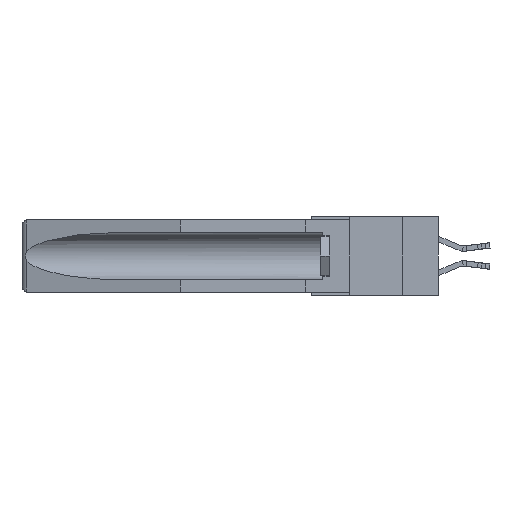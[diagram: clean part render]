
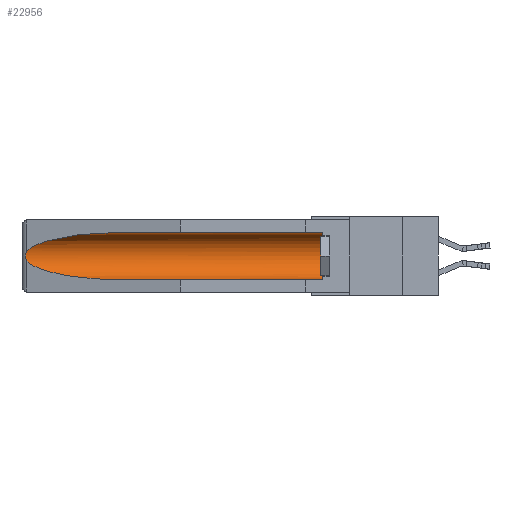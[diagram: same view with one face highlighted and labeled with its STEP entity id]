
A CAD part, left-side view. The second image highlights one B-rep face of the part: STEP entity #22956.
In plain terms, the highlighted cylindrical face has radius 2.857 mm (diameter 5.715 mm), a partial arc.
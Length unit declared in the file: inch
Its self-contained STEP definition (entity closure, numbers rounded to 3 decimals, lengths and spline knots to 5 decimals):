
#512 = CARTESIAN_POINT ( 'NONE',  ( 0.26654, 1.53092, -0.15636 ) ) ;
#1495 = B_SPLINE_CURVE_WITH_KNOTS ( 'NONE', 3,
 ( #16383, #3281, #512, #19023, #21799, #3167, #21676, #3513, #32381, #22036 ),
 .UNSPECIFIED., .F., .F.,
 ( 4, 2, 2, 2, 4 ),
 ( 0., 0.00029, 0.00058, 0.00087, 0.00117 ),
 .UNSPECIFIED. ) ;
#1507 = CARTESIAN_POINT ( 'NONE',  ( 0.155, 0.126, -0.284 ) ) ;
#3167 = CARTESIAN_POINT ( 'NONE',  ( 0.2675, 1.53308, -0.17534 ) ) ;
#3248 = ORIENTED_EDGE ( 'NONE', *, *, #4198, .T. ) ;
#3281 = CARTESIAN_POINT ( 'NONE',  ( 0.26597, 1.52961, -0.15275 ) ) ;
#3391 =( BOUNDED_CURVE ( )  B_SPLINE_CURVE ( 3, ( #12458, #20288, #14993, #14761 ),
 .UNSPECIFIED., .F., .F. ) 
 B_SPLINE_CURVE_WITH_KNOTS ( ( 4, 4 ),
 ( 4.71239, 6.08839 ),
 .UNSPECIFIED. ) 
 CURVE ( )  GEOMETRIC_REPRESENTATION_ITEM ( )  RATIONAL_B_SPLINE_CURVE ( ( 1., 0.848, 0.848, 1. ) ) 
 REPRESENTATION_ITEM ( '' )  );
#3513 = CARTESIAN_POINT ( 'NONE',  ( 0.26655, 1.53094, -0.18657 ) ) ;
#4198 = EDGE_CURVE ( 'NONE', #24264, #15931, #30699, .T. ) ;
#4644 = ORIENTED_EDGE ( 'NONE', *, *, #19632, .T. ) ;
#4700 = ORIENTED_EDGE ( 'NONE', *, *, #30268, .T. ) ;
#4948 = VERTEX_POINT ( 'NONE', #6876 ) ;
#5001 = VECTOR ( 'NONE', #31620, 39.37008 ) ;
#5526 = VERTEX_POINT ( 'NONE', #1507 ) ;
#6672 = CARTESIAN_POINT ( 'NONE',  ( 0.26537, 1.52718, -0.19328 ) ) ;
#6876 = CARTESIAN_POINT ( 'NONE',  ( 0.155, 0.126, -0.059 ) ) ;
#7741 = LINE ( 'NONE', #17487, #27625 ) ;
#8309 = CARTESIAN_POINT ( 'NONE',  ( 0.25451, 1.48313, -0.24835 ) ) ;
#10402 = LINE ( 'NONE', #29444, #5001 ) ;
#10989 = CARTESIAN_POINT ( 'NONE',  ( 0.155, 1.07973, -0.284 ) ) ;
#11816 = AXIS2_PLACEMENT_3D ( 'NONE', #27586, #27694, #30078 ) ;
#12458 = CARTESIAN_POINT ( 'NONE',  ( 0.155, 1.07973, -0.059 ) ) ;
#12667 = VERTEX_POINT ( 'NONE', #12858 ) ;
#12858 = CARTESIAN_POINT ( 'NONE',  ( 0.26537, 1.52718, -0.14972 ) ) ;
#12925 = CARTESIAN_POINT ( 'NONE',  ( 0.155, 0.126, -0.1715 ) ) ;
#14761 = CARTESIAN_POINT ( 'NONE',  ( 0.26537, 1.52718, -0.14972 ) ) ;
#14993 = CARTESIAN_POINT ( 'NONE',  ( 0.25451, 1.48313, -0.09465 ) ) ;
#15931 = VERTEX_POINT ( 'NONE', #20231 ) ;
#16383 = CARTESIAN_POINT ( 'NONE',  ( 0.26537, 1.52718, -0.14972 ) ) ;
#16407 = CARTESIAN_POINT ( 'NONE',  ( 0.21114, 1.30732, -0.284 ) ) ;
#16977 = EDGE_CURVE ( 'NONE', #5526, #15931, #10402, .T. ) ;
#17487 = CARTESIAN_POINT ( 'NONE',  ( 0.155, -0.30754, -0.059 ) ) ;
#19023 = CARTESIAN_POINT ( 'NONE',  ( 0.2673, 1.5327, -0.16383 ) ) ;
#19632 = EDGE_CURVE ( 'NONE', #4948, #30372, #7741, .T. ) ;
#20231 = CARTESIAN_POINT ( 'NONE',  ( 0.155, 1.07973, -0.284 ) ) ;
#20288 = CARTESIAN_POINT ( 'NONE',  ( 0.21114, 1.30732, -0.059 ) ) ;
#21014 = AXIS2_PLACEMENT_3D ( 'NONE', #12925, #26079, #31247 ) ;
#21676 = CARTESIAN_POINT ( 'NONE',  ( 0.2673, 1.53269, -0.17917 ) ) ;
#21703 = CARTESIAN_POINT ( 'NONE',  ( 0.26537, 1.52718, -0.19328 ) ) ;
#21799 = CARTESIAN_POINT ( 'NONE',  ( 0.2675, 1.53308, -0.16763 ) ) ;
#22036 = CARTESIAN_POINT ( 'NONE',  ( 0.26537, 1.52718, -0.19328 ) ) ;
#22956 = ADVANCED_FACE ( 'NONE', ( #33935 ), #23648, .F. ) ;
#23648 = CYLINDRICAL_SURFACE ( 'NONE', #11816, 0.1125 ) ;
#24264 = VERTEX_POINT ( 'NONE', #6672 ) ;
#26079 = DIRECTION ( 'NONE',  ( 0., -1., 0. ) ) ;
#26179 = CARTESIAN_POINT ( 'NONE',  ( 0.155, 1.07973, -0.059 ) ) ;
#26290 = ORIENTED_EDGE ( 'NONE', *, *, #33363, .T. ) ;
#26767 = CIRCLE ( 'NONE', #21014, 0.1125 ) ;
#27586 = CARTESIAN_POINT ( 'NONE',  ( 0.155, -0.30754, -0.1715 ) ) ;
#27625 = VECTOR ( 'NONE', #30380, 39.37008 ) ;
#27694 = DIRECTION ( 'NONE',  ( 0., 1., 0. ) ) ;
#28148 = EDGE_CURVE ( 'NONE', #30372, #12667, #3391, .T. ) ;
#29419 = ORIENTED_EDGE ( 'NONE', *, *, #28148, .T. ) ;
#29444 = CARTESIAN_POINT ( 'NONE',  ( 0.155, -0.30754, -0.284 ) ) ;
#30078 = DIRECTION ( 'NONE',  ( 0., 0., 1. ) ) ;
#30268 = EDGE_CURVE ( 'NONE', #5526, #4948, #26767, .T. ) ;
#30372 = VERTEX_POINT ( 'NONE', #26179 ) ;
#30380 = DIRECTION ( 'NONE',  ( 0., 1., 0. ) ) ;
#30699 =( BOUNDED_CURVE ( )  B_SPLINE_CURVE ( 3, ( #21703, #8309, #16407, #10989 ),
 .UNSPECIFIED., .F., .F. ) 
 B_SPLINE_CURVE_WITH_KNOTS ( ( 4, 4 ),
 ( 0.1948, 1.5708 ),
 .UNSPECIFIED. ) 
 CURVE ( )  GEOMETRIC_REPRESENTATION_ITEM ( )  RATIONAL_B_SPLINE_CURVE ( ( 1., 0.848, 0.848, 1. ) ) 
 REPRESENTATION_ITEM ( '' )  );
#31247 = DIRECTION ( 'NONE',  ( 0., 0., 1. ) ) ;
#31620 = DIRECTION ( 'NONE',  ( 0., 1., 0. ) ) ;
#32381 = CARTESIAN_POINT ( 'NONE',  ( 0.26597, 1.5296, -0.19026 ) ) ;
#32805 = EDGE_LOOP ( 'NONE', ( #29419, #26290, #3248, #33967, #4700, #4644 ) ) ;
#33363 = EDGE_CURVE ( 'NONE', #12667, #24264, #1495, .T. ) ;
#33935 = FACE_OUTER_BOUND ( 'NONE', #32805, .T. ) ;
#33967 = ORIENTED_EDGE ( 'NONE', *, *, #16977, .F. ) ;
